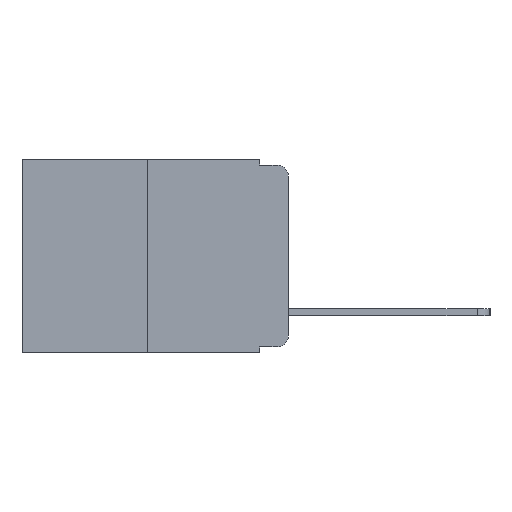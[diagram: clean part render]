
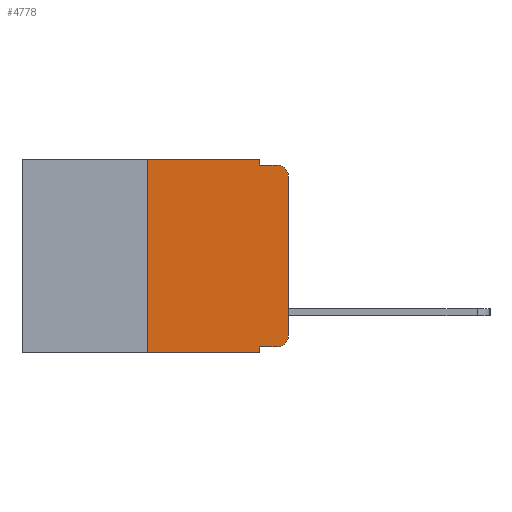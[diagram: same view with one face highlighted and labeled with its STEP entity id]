
A CAD part, left-side view. The second image highlights one B-rep face of the part: STEP entity #4778.
In plain terms, the highlighted planar face has unit normal (-1, 0, 0).
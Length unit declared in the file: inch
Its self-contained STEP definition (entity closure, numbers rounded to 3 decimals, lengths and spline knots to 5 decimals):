
#72 = VERTEX_POINT ( 'NONE', #10882 ) ;
#443 = DIRECTION ( 'NONE',  ( 0., 0., 1. ) ) ;
#465 = ORIENTED_EDGE ( 'NONE', *, *, #8476, .T. ) ;
#479 = CARTESIAN_POINT ( 'NONE',  ( 0., 0.051, -0.343 ) ) ;
#531 = ORIENTED_EDGE ( 'NONE', *, *, #7245, .T. ) ;
#590 = CARTESIAN_POINT ( 'NONE',  ( 0., 0.473, 0. ) ) ;
#652 = VECTOR ( 'NONE', #11532, 39.37008 ) ;
#860 = DIRECTION ( 'NONE',  ( -1., 0., 0. ) ) ;
#1308 = EDGE_LOOP ( 'NONE', ( #11147, #9309, #7860, #1503, #2364, #8370, #2581, #2870, #465, #531 ) ) ;
#1503 = ORIENTED_EDGE ( 'NONE', *, *, #11577, .F. ) ;
#2024 = VERTEX_POINT ( 'NONE', #479 ) ;
#2106 = LINE ( 'NONE', #2521, #9512 ) ;
#2364 = ORIENTED_EDGE ( 'NONE', *, *, #8523, .F. ) ;
#2479 = CARTESIAN_POINT ( 'NONE',  ( 0., 0., -0.03 ) ) ;
#2521 = CARTESIAN_POINT ( 'NONE',  ( 0., 0.25, 0. ) ) ;
#2529 = CARTESIAN_POINT ( 'NONE',  ( 0., 0., -0.313 ) ) ;
#2581 = ORIENTED_EDGE ( 'NONE', *, *, #3775, .T. ) ;
#2870 = ORIENTED_EDGE ( 'NONE', *, *, #10302, .F. ) ;
#2892 = CARTESIAN_POINT ( 'NONE',  ( 0., 0.25, -0.343 ) ) ;
#3124 = DIRECTION ( 'NONE',  ( 1., 0., 0. ) ) ;
#3142 = VERTEX_POINT ( 'NONE', #2529 ) ;
#3393 = CARTESIAN_POINT ( 'NONE',  ( 0., 0.051, -0.333 ) ) ;
#3469 = CARTESIAN_POINT ( 'NONE',  ( 0., 0.473, -0.343 ) ) ;
#3493 = DIRECTION ( 'NONE',  ( 0., 0., -1. ) ) ;
#3775 = EDGE_CURVE ( 'NONE', #4017, #2024, #8108, .T. ) ;
#3846 = VERTEX_POINT ( 'NONE', #3393 ) ;
#4017 = VERTEX_POINT ( 'NONE', #2892 ) ;
#4231 = AXIS2_PLACEMENT_3D ( 'NONE', #11351, #5799, #12286 ) ;
#4778 = ADVANCED_FACE ( 'NONE', ( #9796 ), #7034, .F. ) ;
#4808 = VERTEX_POINT ( 'NONE', #9846 ) ;
#4979 = CARTESIAN_POINT ( 'NONE',  ( 0., 0., 0. ) ) ;
#5359 = AXIS2_PLACEMENT_3D ( 'NONE', #11639, #3124, #9809 ) ;
#5549 = VERTEX_POINT ( 'NONE', #7174 ) ;
#5622 = VECTOR ( 'NONE', #9189, 39.37008 ) ;
#5799 = DIRECTION ( 'NONE',  ( -1., 0., 0. ) ) ;
#5819 = DIRECTION ( 'NONE',  ( 0., -1., 0. ) ) ;
#6640 = DIRECTION ( 'NONE',  ( 0., -1., 0. ) ) ;
#6883 = CARTESIAN_POINT ( 'NONE',  ( 0., 0.02, -0.313 ) ) ;
#6977 = VECTOR ( 'NONE', #6640, 39.37008 ) ;
#7016 = CIRCLE ( 'NONE', #9757, 0.02 ) ;
#7034 = PLANE ( 'NONE',  #5359 ) ;
#7174 = CARTESIAN_POINT ( 'NONE',  ( 0., 0.25, 0. ) ) ;
#7245 = EDGE_CURVE ( 'NONE', #10410, #3142, #7016, .T. ) ;
#7372 = CARTESIAN_POINT ( 'NONE',  ( 0., 0.051, 0. ) ) ;
#7799 = DIRECTION ( 'NONE',  ( 0., 0., -1. ) ) ;
#7860 = ORIENTED_EDGE ( 'NONE', *, *, #12188, .F. ) ;
#7875 = VECTOR ( 'NONE', #9231, 39.37008 ) ;
#7888 = CIRCLE ( 'NONE', #4231, 0.02 ) ;
#8044 = LINE ( 'NONE', #7372, #8338 ) ;
#8108 = LINE ( 'NONE', #3469, #5622 ) ;
#8128 = LINE ( 'NONE', #8625, #12453 ) ;
#8338 = VECTOR ( 'NONE', #3493, 39.37008 ) ;
#8370 = ORIENTED_EDGE ( 'NONE', *, *, #10932, .F. ) ;
#8476 = EDGE_CURVE ( 'NONE', #3846, #10410, #8128, .T. ) ;
#8523 = EDGE_CURVE ( 'NONE', #5549, #10465, #9437, .T. ) ;
#8625 = CARTESIAN_POINT ( 'NONE',  ( 0., 0.051, -0.333 ) ) ;
#9022 = VERTEX_POINT ( 'NONE', #2479 ) ;
#9121 = VECTOR ( 'NONE', #12058, 39.37008 ) ;
#9189 = DIRECTION ( 'NONE',  ( 0., -1., 0. ) ) ;
#9231 = DIRECTION ( 'NONE',  ( 0., -1., 0. ) ) ;
#9309 = ORIENTED_EDGE ( 'NONE', *, *, #11789, .T. ) ;
#9437 = LINE ( 'NONE', #590, #6977 ) ;
#9512 = VECTOR ( 'NONE', #443, 39.37008 ) ;
#9684 = LINE ( 'NONE', #11107, #9121 ) ;
#9757 = AXIS2_PLACEMENT_3D ( 'NONE', #6883, #860, #7799 ) ;
#9796 = FACE_OUTER_BOUND ( 'NONE', #1308, .T. ) ;
#9809 = DIRECTION ( 'NONE',  ( 0., 0., -1. ) ) ;
#9846 = CARTESIAN_POINT ( 'NONE',  ( 0., 0.02, -0.01 ) ) ;
#9957 = EDGE_CURVE ( 'NONE', #3142, #9022, #10967, .T. ) ;
#10302 = EDGE_CURVE ( 'NONE', #3846, #2024, #9684, .T. ) ;
#10315 = LINE ( 'NONE', #11006, #7875 ) ;
#10410 = VERTEX_POINT ( 'NONE', #11229 ) ;
#10465 = VERTEX_POINT ( 'NONE', #11346 ) ;
#10882 = CARTESIAN_POINT ( 'NONE',  ( 0., 0.051, -0.01 ) ) ;
#10932 = EDGE_CURVE ( 'NONE', #4017, #5549, #2106, .T. ) ;
#10967 = LINE ( 'NONE', #4979, #652 ) ;
#11006 = CARTESIAN_POINT ( 'NONE',  ( 0., 0.051, -0.01 ) ) ;
#11107 = CARTESIAN_POINT ( 'NONE',  ( 0., 0.051, 0. ) ) ;
#11147 = ORIENTED_EDGE ( 'NONE', *, *, #9957, .T. ) ;
#11229 = CARTESIAN_POINT ( 'NONE',  ( 0., 0.02, -0.333 ) ) ;
#11346 = CARTESIAN_POINT ( 'NONE',  ( 0., 0.051, 0. ) ) ;
#11351 = CARTESIAN_POINT ( 'NONE',  ( 0., 0.02, -0.03 ) ) ;
#11532 = DIRECTION ( 'NONE',  ( 0., 0., 1. ) ) ;
#11577 = EDGE_CURVE ( 'NONE', #10465, #72, #8044, .T. ) ;
#11639 = CARTESIAN_POINT ( 'NONE',  ( 0., 0.473, 0. ) ) ;
#11789 = EDGE_CURVE ( 'NONE', #9022, #4808, #7888, .T. ) ;
#12058 = DIRECTION ( 'NONE',  ( 0., 0., -1. ) ) ;
#12188 = EDGE_CURVE ( 'NONE', #72, #4808, #10315, .T. ) ;
#12286 = DIRECTION ( 'NONE',  ( 0., 0., -1. ) ) ;
#12453 = VECTOR ( 'NONE', #5819, 39.37008 ) ;
